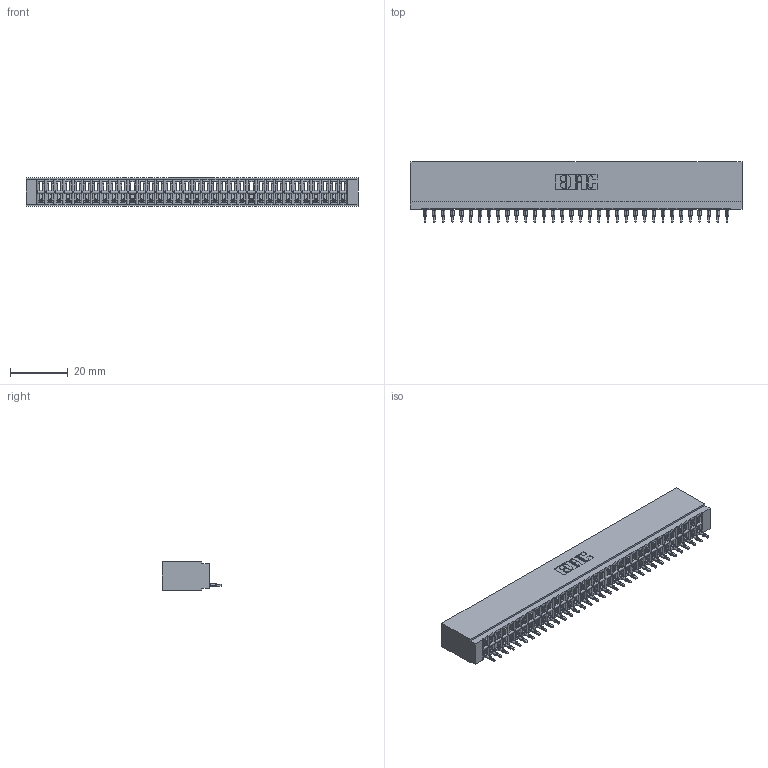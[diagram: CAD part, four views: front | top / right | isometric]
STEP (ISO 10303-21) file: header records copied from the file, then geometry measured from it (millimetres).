
FILE_DESCRIPTION (( 'STEP AP203' ), '1' );
FILE_NAME ('746-034-520-501.STEP', '2026-03-04T13:52:32', ( '' ), ( '' ), 'SwSTEP 2.0', 'SolidWorks 2023', '' );
FILE_SCHEMA (( 'CONFIG_CONTROL_DESIGN' ));
Length unit declared in the file: millimetre
Products named in the file (3): 746-292-001_520; 746-034-520-501; 746 Part_.340 Slot Depth - 01
Assembly tree (35 placements, depth 2):
  746-034-520-501
    746 Part_.340 Slot Depth - 01
    746-292-001_520  x34
Bounding box: 115.19 x 20.82 x 9.91 mm (x, y, z)
Volume: 12929.2 mm3; surface area: 17062.4 mm2
Topology: 35 solids, 35 shells, 3769 faces, 10701 edges, 6873 vertices
Faces by surface type: plane 2197, cylinder 688, bspline 680, torus 204
Entity records: 52505 total; most frequent: CARTESIAN_POINT 10691, ORIENTED_EDGE 9192, DIRECTION 7620, EDGE_CURVE 4596, LINE 4072, VECTOR 4072, VERTEX_POINT 3045, AXIS2_PLACEMENT_3D 1774
